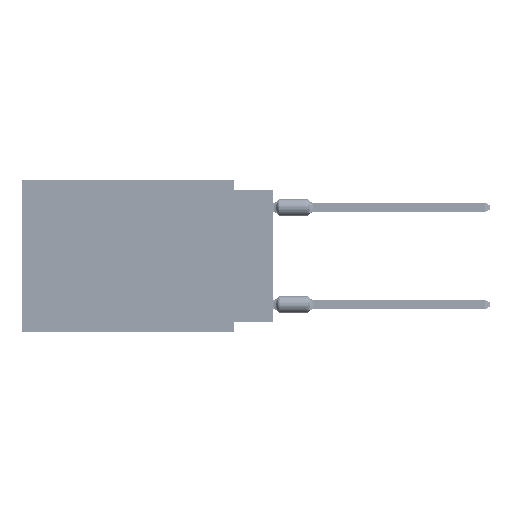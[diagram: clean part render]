
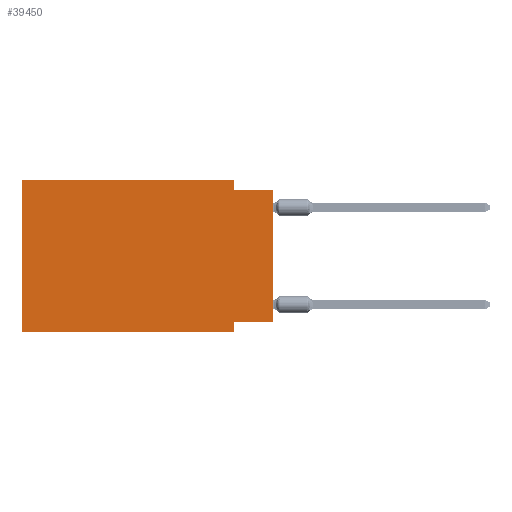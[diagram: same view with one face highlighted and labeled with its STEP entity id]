
A CAD part, left-side view. The second image highlights one B-rep face of the part: STEP entity #39450.
In plain terms, the highlighted planar face has unit normal (-1, 0, 0).
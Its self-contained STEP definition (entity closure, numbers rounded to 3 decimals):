
#162 = LINE ( 'NONE', #45757, #6367 ) ;
#180 = CARTESIAN_POINT ( 'NONE',  ( 0., 2.54, -9.906 ) ) ;
#1617 = CARTESIAN_POINT ( 'NONE',  ( 0., 0., -9.271 ) ) ;
#4111 = LINE ( 'NONE', #82274, #80012 ) ;
#4394 = ORIENTED_EDGE ( 'NONE', *, *, #54060, .F. ) ;
#5382 = CARTESIAN_POINT ( 'NONE',  ( 0., 2.54, -9.271 ) ) ;
#5719 = CARTESIAN_POINT ( 'NONE',  ( 0., 0., -0.635 ) ) ;
#5889 = VERTEX_POINT ( 'NONE', #22909 ) ;
#6367 = VECTOR ( 'NONE', #84842, 1000. ) ;
#8786 = VECTOR ( 'NONE', #31792, 1000. ) ;
#9344 = CARTESIAN_POINT ( 'NONE',  ( 0., 16.383, -9.906 ) ) ;
#11582 = CARTESIAN_POINT ( 'NONE',  ( 0., 2.54, 0. ) ) ;
#12731 = DIRECTION ( 'NONE',  ( 0., 0., -1. ) ) ;
#15128 = CARTESIAN_POINT ( 'NONE',  ( 0., 16.383, -9.906 ) ) ;
#15416 = DIRECTION ( 'NONE',  ( 1., 0., 0. ) ) ;
#17643 = ORIENTED_EDGE ( 'NONE', *, *, #84751, .T. ) ;
#21227 = LINE ( 'NONE', #15128, #72970 ) ;
#22909 = CARTESIAN_POINT ( 'NONE',  ( 0., 0., -0.635 ) ) ;
#24947 = ORIENTED_EDGE ( 'NONE', *, *, #56038, .F. ) ;
#26406 = DIRECTION ( 'NONE',  ( 0., -1., 0. ) ) ;
#26588 = VERTEX_POINT ( 'NONE', #9344 ) ;
#26692 = ORIENTED_EDGE ( 'NONE', *, *, #52763, .F. ) ;
#28040 = CARTESIAN_POINT ( 'NONE',  ( 0., 16.383, 0. ) ) ;
#28889 = PLANE ( 'NONE',  #54960 ) ;
#29308 = DIRECTION ( 'NONE',  ( 0., 0., -1. ) ) ;
#30595 = DIRECTION ( 'NONE',  ( 0., 0., 1. ) ) ;
#31792 = DIRECTION ( 'NONE',  ( 0., -1., 0. ) ) ;
#33146 = CARTESIAN_POINT ( 'NONE',  ( 0., 2.54, 0. ) ) ;
#33203 = EDGE_CURVE ( 'NONE', #43518, #52594, #85268, .T. ) ;
#34249 = VERTEX_POINT ( 'NONE', #38800 ) ;
#34976 = ORIENTED_EDGE ( 'NONE', *, *, #72251, .F. ) ;
#38121 = LINE ( 'NONE', #71976, #85364 ) ;
#38529 = ORIENTED_EDGE ( 'NONE', *, *, #75077, .T. ) ;
#38732 = LINE ( 'NONE', #5719, #8786 ) ;
#38800 = CARTESIAN_POINT ( 'NONE',  ( 0., 2.54, -0.635 ) ) ;
#39450 = ADVANCED_FACE ( 'NONE', ( #61457 ), #28889, .F. ) ;
#41039 = VERTEX_POINT ( 'NONE', #11582 ) ;
#42772 = ORIENTED_EDGE ( 'NONE', *, *, #56155, .F. ) ;
#43518 = VERTEX_POINT ( 'NONE', #5382 ) ;
#44723 = ORIENTED_EDGE ( 'NONE', *, *, #33203, .F. ) ;
#44907 = VECTOR ( 'NONE', #26406, 1000. ) ;
#45757 = CARTESIAN_POINT ( 'NONE',  ( 0., 0., -9.271 ) ) ;
#47656 = VERTEX_POINT ( 'NONE', #74997 ) ;
#47697 = DIRECTION ( 'NONE',  ( 0., -1., 0. ) ) ;
#52594 = VERTEX_POINT ( 'NONE', #180 ) ;
#52763 = EDGE_CURVE ( 'NONE', #34249, #5889, #38732, .T. ) ;
#54060 = EDGE_CURVE ( 'NONE', #47656, #41039, #79796, .T. ) ;
#54960 = AXIS2_PLACEMENT_3D ( 'NONE', #28040, #15416, #29308 ) ;
#56038 = EDGE_CURVE ( 'NONE', #26588, #47656, #4111, .T. ) ;
#56155 = EDGE_CURVE ( 'NONE', #74101, #43518, #162, .T. ) ;
#58953 = DIRECTION ( 'NONE',  ( 0., 0., 1. ) ) ;
#60063 = DIRECTION ( 'NONE',  ( 0., 0., -1. ) ) ;
#61457 = FACE_OUTER_BOUND ( 'NONE', #70662, .T. ) ;
#66585 = CARTESIAN_POINT ( 'NONE',  ( 0., 2.54, -9.906 ) ) ;
#70662 = EDGE_LOOP ( 'NONE', ( #38529, #26692, #34976, #4394, #24947, #17643, #44723, #42772 ) ) ;
#71976 = CARTESIAN_POINT ( 'NONE',  ( 0., 0., 0. ) ) ;
#72251 = EDGE_CURVE ( 'NONE', #41039, #34249, #84832, .T. ) ;
#72970 = VECTOR ( 'NONE', #47697, 1000. ) ;
#74101 = VERTEX_POINT ( 'NONE', #1617 ) ;
#74948 = VECTOR ( 'NONE', #60063, 1000. ) ;
#74997 = CARTESIAN_POINT ( 'NONE',  ( 0., 16.383, 0. ) ) ;
#75077 = EDGE_CURVE ( 'NONE', #74101, #5889, #38121, .T. ) ;
#78093 = VECTOR ( 'NONE', #12731, 1000. ) ;
#78497 = CARTESIAN_POINT ( 'NONE',  ( 0., 16.383, 0. ) ) ;
#79796 = LINE ( 'NONE', #78497, #44907 ) ;
#80012 = VECTOR ( 'NONE', #30595, 1000. ) ;
#82274 = CARTESIAN_POINT ( 'NONE',  ( 0., 16.383, 0. ) ) ;
#84751 = EDGE_CURVE ( 'NONE', #26588, #52594, #21227, .T. ) ;
#84832 = LINE ( 'NONE', #33146, #78093 ) ;
#84842 = DIRECTION ( 'NONE',  ( 0., 1., 0. ) ) ;
#85268 = LINE ( 'NONE', #66585, #74948 ) ;
#85364 = VECTOR ( 'NONE', #58953, 1000. ) ;
